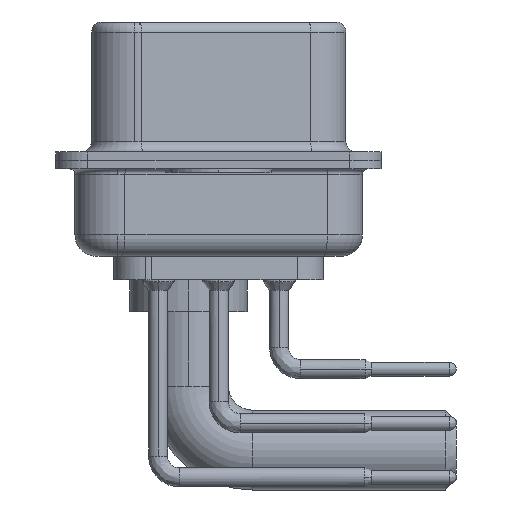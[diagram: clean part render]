
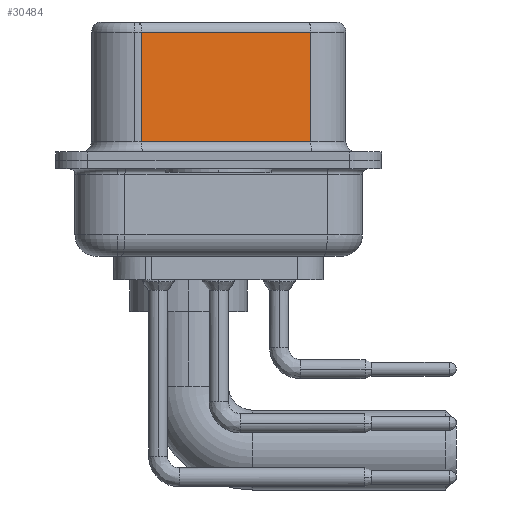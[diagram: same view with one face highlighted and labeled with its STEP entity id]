
A CAD part, left-side view. The second image highlights one B-rep face of the part: STEP entity #30484.
In plain terms, the highlighted planar face has unit normal (-0.985, -0.174, 0).
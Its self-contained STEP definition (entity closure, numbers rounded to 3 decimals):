
#113 = LINE ( 'NONE', #21720, #16178 ) ;
#445 = EDGE_LOOP ( 'NONE', ( #9440, #21162, #4210, #5055 ) ) ;
#3964 = EDGE_CURVE ( 'NONE', #10502, #14280, #113, .T. ) ;
#4210 = ORIENTED_EDGE ( 'NONE', *, *, #27624, .T. ) ;
#5024 = FACE_OUTER_BOUND ( 'NONE', #445, .T. ) ;
#5055 = ORIENTED_EDGE ( 'NONE', *, *, #8813, .T. ) ;
#5202 = DIRECTION ( 'NONE',  ( 0.985, 0.174, 0. ) ) ;
#6308 = LINE ( 'NONE', #28466, #23958 ) ;
#8274 = CARTESIAN_POINT ( 'NONE',  ( 5.132, -4.322, 6.52 ) ) ;
#8401 = CARTESIAN_POINT ( 'NONE',  ( 3.73, 3.628, 6.02 ) ) ;
#8750 = CARTESIAN_POINT ( 'NONE',  ( 5.132, -4.322, 0.9 ) ) ;
#8813 = EDGE_CURVE ( 'NONE', #10090, #14280, #6308, .T. ) ;
#9440 = ORIENTED_EDGE ( 'NONE', *, *, #3964, .F. ) ;
#10090 = VERTEX_POINT ( 'NONE', #22507 ) ;
#10502 = VERTEX_POINT ( 'NONE', #13104 ) ;
#11108 = DIRECTION ( 'NONE',  ( 0., 0., -1. ) ) ;
#11482 = LINE ( 'NONE', #33436, #26434 ) ;
#11525 = VECTOR ( 'NONE', #18067, 1000. ) ;
#12498 = CARTESIAN_POINT ( 'NONE',  ( 5.132, -4.322, 6.02 ) ) ;
#13104 = CARTESIAN_POINT ( 'NONE',  ( 5.132, -4.322, 6.02 ) ) ;
#14280 = VERTEX_POINT ( 'NONE', #8750 ) ;
#16178 = VECTOR ( 'NONE', #11108, 1000. ) ;
#18067 = DIRECTION ( 'NONE',  ( -0.174, 0.985, 0. ) ) ;
#21162 = ORIENTED_EDGE ( 'NONE', *, *, #28197, .T. ) ;
#21720 = CARTESIAN_POINT ( 'NONE',  ( 5.132, -4.322, 6.52 ) ) ;
#22495 = AXIS2_PLACEMENT_3D ( 'NONE', #8274, #5202, #32553 ) ;
#22507 = CARTESIAN_POINT ( 'NONE',  ( 3.73, 3.628, 0.9 ) ) ;
#23958 = VECTOR ( 'NONE', #25576, 1000. ) ;
#25576 = DIRECTION ( 'NONE',  ( 0.174, -0.985, 0. ) ) ;
#25912 = VERTEX_POINT ( 'NONE', #8401 ) ;
#26434 = VECTOR ( 'NONE', #28228, 1000. ) ;
#26695 = LINE ( 'NONE', #12498, #11525 ) ;
#27624 = EDGE_CURVE ( 'NONE', #25912, #10090, #11482, .T. ) ;
#28197 = EDGE_CURVE ( 'NONE', #10502, #25912, #26695, .T. ) ;
#28228 = DIRECTION ( 'NONE',  ( 0., 0., -1. ) ) ;
#28466 = CARTESIAN_POINT ( 'NONE',  ( 5.132, -4.322, 0.9 ) ) ;
#30484 = ADVANCED_FACE ( 'NONE', ( #5024 ), #32911, .F. ) ;
#32553 = DIRECTION ( 'NONE',  ( -0.174, 0.985, 0. ) ) ;
#32911 = PLANE ( 'NONE',  #22495 ) ;
#33436 = CARTESIAN_POINT ( 'NONE',  ( 3.73, 3.628, 6.52 ) ) ;
